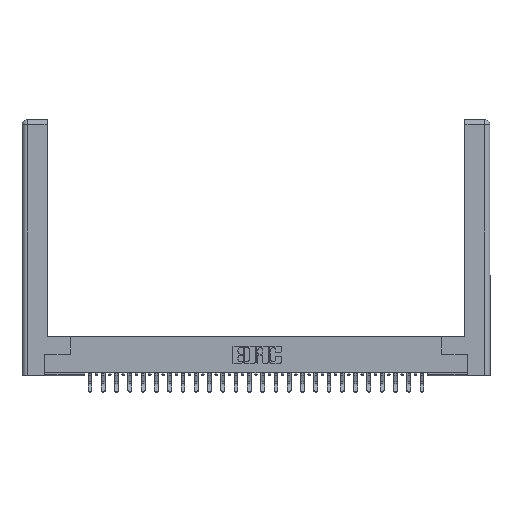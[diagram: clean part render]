
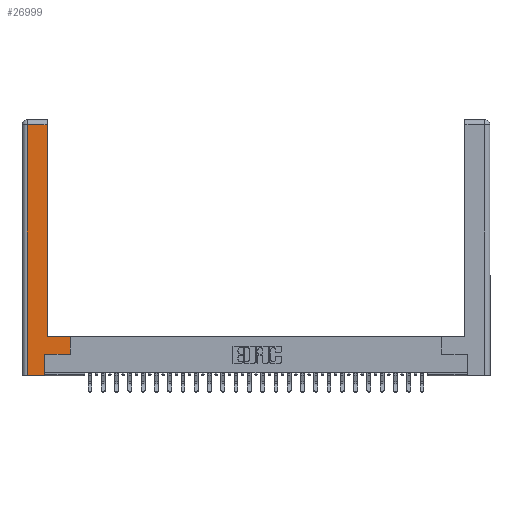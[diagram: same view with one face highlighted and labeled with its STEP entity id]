
A CAD part, top view. The second image highlights one B-rep face of the part: STEP entity #26999.
In plain terms, the highlighted planar face has unit normal (0, 0, 1).
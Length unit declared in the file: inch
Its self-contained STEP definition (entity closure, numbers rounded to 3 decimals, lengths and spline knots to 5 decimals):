
#1173 = DIRECTION ( 'NONE',  ( 0., 1., 0. ) ) ;
#1864 = ORIENTED_EDGE ( 'NONE', *, *, #11727, .T. ) ;
#2563 = VECTOR ( 'NONE', #13511, 39.37008 ) ;
#2779 = VECTOR ( 'NONE', #6868, 39.37008 ) ;
#2946 = LINE ( 'NONE', #27471, #24091 ) ;
#3809 = ORIENTED_EDGE ( 'NONE', *, *, #26277, .T. ) ;
#5235 = ORIENTED_EDGE ( 'NONE', *, *, #20636, .T. ) ;
#5850 = DIRECTION ( 'NONE',  ( -1., 0., 0. ) ) ;
#6868 = DIRECTION ( 'NONE',  ( 1., 0., 0. ) ) ;
#7734 = CARTESIAN_POINT ( 'NONE',  ( 0.565, 0.245, 0. ) ) ;
#8146 = ORIENTED_EDGE ( 'NONE', *, *, #29947, .T. ) ;
#8767 = DIRECTION ( 'NONE',  ( 0., -1., 0. ) ) ;
#9032 = ORIENTED_EDGE ( 'NONE', *, *, #14399, .T. ) ;
#9221 = DIRECTION ( 'NONE',  ( -1., 0., 0. ) ) ;
#9280 = CARTESIAN_POINT ( 'NONE',  ( 0.295, 2.94, 0. ) ) ;
#9563 = CARTESIAN_POINT ( 'NONE',  ( 0., 0., 0. ) ) ;
#10616 = VECTOR ( 'NONE', #11700, 39.37008 ) ;
#11216 = VECTOR ( 'NONE', #5850, 39.37008 ) ;
#11475 = VERTEX_POINT ( 'NONE', #20730 ) ;
#11639 = VECTOR ( 'NONE', #1173, 39.37008 ) ;
#11700 = DIRECTION ( 'NONE',  ( 0., 1., 0. ) ) ;
#11727 = EDGE_CURVE ( 'NONE', #30403, #24288, #23922, .T. ) ;
#11805 = VERTEX_POINT ( 'NONE', #30060 ) ;
#12019 = DIRECTION ( 'NONE',  ( 0., 0., -1. ) ) ;
#12122 = PLANE ( 'NONE',  #27443 ) ;
#12128 = CARTESIAN_POINT ( 'NONE',  ( 0.265, 0.245, 0. ) ) ;
#13511 = DIRECTION ( 'NONE',  ( 0., 1., 0. ) ) ;
#13629 = EDGE_CURVE ( 'NONE', #24851, #26691, #2946, .T. ) ;
#13694 = VECTOR ( 'NONE', #8767, 39.37008 ) ;
#13812 = CARTESIAN_POINT ( 'NONE',  ( 0.565, 0.45, 0. ) ) ;
#13917 = CARTESIAN_POINT ( 'NONE',  ( 0.0615, 0., 0. ) ) ;
#14376 = CARTESIAN_POINT ( 'NONE',  ( 0.265, 0., 0. ) ) ;
#14399 = EDGE_CURVE ( 'NONE', #26691, #30403, #29155, .T. ) ;
#14878 = EDGE_CURVE ( 'NONE', #24288, #11475, #14994, .T. ) ;
#14897 = CARTESIAN_POINT ( 'NONE',  ( 0.565, 0.45, 0. ) ) ;
#14994 = LINE ( 'NONE', #12128, #10616 ) ;
#15337 = CARTESIAN_POINT ( 'NONE',  ( 0.565, 0.245, 0. ) ) ;
#15358 = LINE ( 'NONE', #28665, #2563 ) ;
#17527 = EDGE_CURVE ( 'NONE', #11475, #20384, #19436, .T. ) ;
#17797 = CARTESIAN_POINT ( 'NONE',  ( 0.0615, 2.94, 0. ) ) ;
#17962 = LINE ( 'NONE', #23993, #11216 ) ;
#18268 = VERTEX_POINT ( 'NONE', #14897 ) ;
#19436 = LINE ( 'NONE', #7734, #26919 ) ;
#20384 = VERTEX_POINT ( 'NONE', #15337 ) ;
#20411 = EDGE_LOOP ( 'NONE', ( #3809, #22221, #9032, #1864, #28193, #28055, #8146, #5235 ) ) ;
#20636 = EDGE_CURVE ( 'NONE', #18268, #11805, #17962, .T. ) ;
#20730 = CARTESIAN_POINT ( 'NONE',  ( 0.265, 0.245, 0. ) ) ;
#21261 = FACE_OUTER_BOUND ( 'NONE', #20411, .T. ) ;
#22221 = ORIENTED_EDGE ( 'NONE', *, *, #13629, .T. ) ;
#22393 = DIRECTION ( 'NONE',  ( -1., 0., 0. ) ) ;
#23200 = DIRECTION ( 'NONE',  ( 1., 0., 0. ) ) ;
#23922 = LINE ( 'NONE', #14376, #2779 ) ;
#23993 = CARTESIAN_POINT ( 'NONE',  ( 0.295, 0.45, 0. ) ) ;
#24091 = VECTOR ( 'NONE', #22393, 39.37008 ) ;
#24288 = VERTEX_POINT ( 'NONE', #32645 ) ;
#24851 = VERTEX_POINT ( 'NONE', #9280 ) ;
#25483 = LINE ( 'NONE', #13812, #11639 ) ;
#26277 = EDGE_CURVE ( 'NONE', #11805, #24851, #15358, .T. ) ;
#26691 = VERTEX_POINT ( 'NONE', #17797 ) ;
#26919 = VECTOR ( 'NONE', #23200, 39.37008 ) ;
#26999 = ADVANCED_FACE ( 'NONE', ( #21261 ), #12122, .F. ) ;
#27443 = AXIS2_PLACEMENT_3D ( 'NONE', #9563, #12019, #9221 ) ;
#27471 = CARTESIAN_POINT ( 'NONE',  ( 0.0615, 2.94, 0. ) ) ;
#28055 = ORIENTED_EDGE ( 'NONE', *, *, #17527, .T. ) ;
#28193 = ORIENTED_EDGE ( 'NONE', *, *, #14878, .T. ) ;
#28665 = CARTESIAN_POINT ( 'NONE',  ( 0.295, 3., 0. ) ) ;
#29155 = LINE ( 'NONE', #13917, #13694 ) ;
#29947 = EDGE_CURVE ( 'NONE', #20384, #18268, #25483, .T. ) ;
#30060 = CARTESIAN_POINT ( 'NONE',  ( 0.295, 0.45, 0. ) ) ;
#30403 = VERTEX_POINT ( 'NONE', #32705 ) ;
#32645 = CARTESIAN_POINT ( 'NONE',  ( 0.265, 0., 0. ) ) ;
#32705 = CARTESIAN_POINT ( 'NONE',  ( 0.0615, 0., 0. ) ) ;
